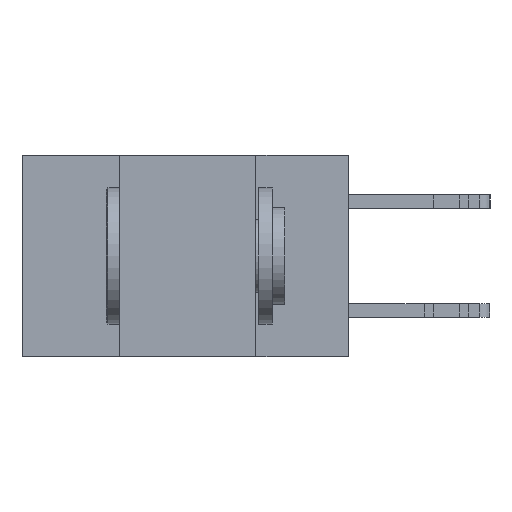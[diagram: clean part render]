
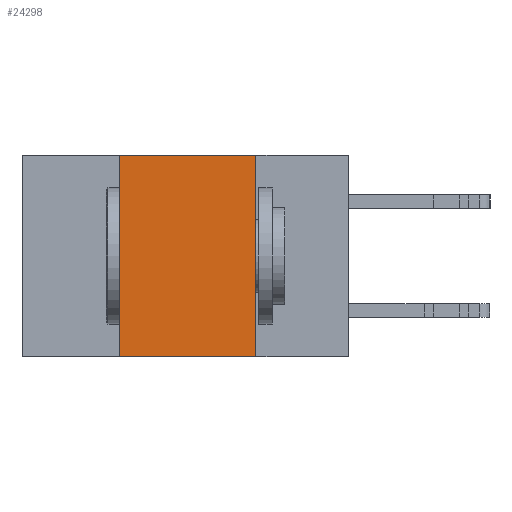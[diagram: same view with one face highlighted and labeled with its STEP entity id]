
A CAD part, left-side view. The second image highlights one B-rep face of the part: STEP entity #24298.
In plain terms, the highlighted planar face has unit normal (-1, 0, 0).
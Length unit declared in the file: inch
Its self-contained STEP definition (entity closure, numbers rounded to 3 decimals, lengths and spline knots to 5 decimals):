
#24 = EDGE_CURVE ( 'NONE', #1613, #18675, #9256, .T. ) ;
#239 = CARTESIAN_POINT ( 'NONE',  ( 0., 0.6, -0.37 ) ) ;
#1527 = DIRECTION ( 'NONE',  ( 1., 0., 0. ) ) ;
#1613 = VERTEX_POINT ( 'NONE', #15380 ) ;
#2658 = LINE ( 'NONE', #239, #25306 ) ;
#2810 = CARTESIAN_POINT ( 'NONE',  ( 0., 0.42, -0.37 ) ) ;
#5122 = CARTESIAN_POINT ( 'NONE',  ( 0., 0.17, -0.37 ) ) ;
#7975 = DIRECTION ( 'NONE',  ( 0., 0., -1. ) ) ;
#8867 = CARTESIAN_POINT ( 'NONE',  ( 0., 0.17, -0.37 ) ) ;
#8902 = LINE ( 'NONE', #25615, #15570 ) ;
#9112 = EDGE_CURVE ( 'NONE', #1613, #15520, #2658, .T. ) ;
#9256 = LINE ( 'NONE', #2810, #25382 ) ;
#9389 = DIRECTION ( 'NONE',  ( 0., -1., 0. ) ) ;
#10016 = VECTOR ( 'NONE', #17617, 39.37008 ) ;
#11419 = CARTESIAN_POINT ( 'NONE',  ( 0., 0.17, 0. ) ) ;
#11541 = DIRECTION ( 'NONE',  ( 0., 0., 1. ) ) ;
#12356 = AXIS2_PLACEMENT_3D ( 'NONE', #18729, #1527, #7975 ) ;
#13297 = EDGE_LOOP ( 'NONE', ( #18358, #20188, #26533, #21600 ) ) ;
#15291 = EDGE_CURVE ( 'NONE', #18675, #27658, #8902, .T. ) ;
#15380 = CARTESIAN_POINT ( 'NONE',  ( 0., 0.42, -0.37 ) ) ;
#15520 = VERTEX_POINT ( 'NONE', #5122 ) ;
#15570 = VECTOR ( 'NONE', #23889, 39.37008 ) ;
#17617 = DIRECTION ( 'NONE',  ( 0., 0., -1. ) ) ;
#18096 = CARTESIAN_POINT ( 'NONE',  ( 0., 0.42, 0. ) ) ;
#18358 = ORIENTED_EDGE ( 'NONE', *, *, #20930, .F. ) ;
#18675 = VERTEX_POINT ( 'NONE', #18096 ) ;
#18729 = CARTESIAN_POINT ( 'NONE',  ( 0., 0.6, 0. ) ) ;
#20188 = ORIENTED_EDGE ( 'NONE', *, *, #15291, .F. ) ;
#20732 = FACE_OUTER_BOUND ( 'NONE', #13297, .T. ) ;
#20930 = EDGE_CURVE ( 'NONE', #27658, #15520, #28202, .T. ) ;
#21600 = ORIENTED_EDGE ( 'NONE', *, *, #9112, .T. ) ;
#23889 = DIRECTION ( 'NONE',  ( 0., -1., 0. ) ) ;
#24298 = ADVANCED_FACE ( 'NONE', ( #20732 ), #27725, .F. ) ;
#25306 = VECTOR ( 'NONE', #9389, 39.37008 ) ;
#25382 = VECTOR ( 'NONE', #11541, 39.37008 ) ;
#25615 = CARTESIAN_POINT ( 'NONE',  ( 0., 0.6, 0. ) ) ;
#26533 = ORIENTED_EDGE ( 'NONE', *, *, #24, .F. ) ;
#27658 = VERTEX_POINT ( 'NONE', #11419 ) ;
#27725 = PLANE ( 'NONE',  #12356 ) ;
#28202 = LINE ( 'NONE', #8867, #10016 ) ;
